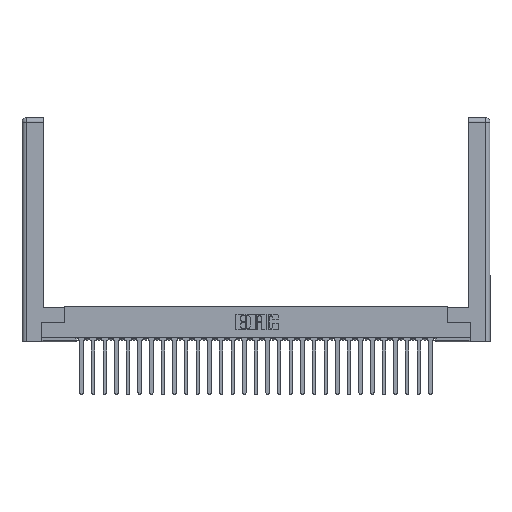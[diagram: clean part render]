
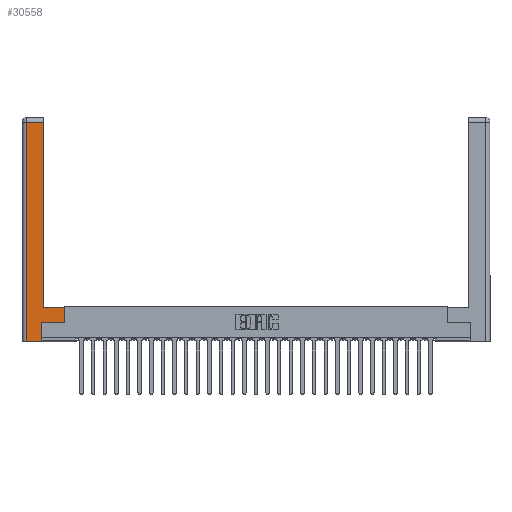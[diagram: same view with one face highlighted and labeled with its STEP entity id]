
A CAD part, top view. The second image highlights one B-rep face of the part: STEP entity #30558.
In plain terms, the highlighted planar face has unit normal (0, 0, 1).
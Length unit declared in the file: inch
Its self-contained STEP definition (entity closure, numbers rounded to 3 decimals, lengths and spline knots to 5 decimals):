
#816 = EDGE_CURVE ( 'NONE', #7851, #13557, #26790, .T. ) ;
#1370 = VECTOR ( 'NONE', #30396, 39.37008 ) ;
#1423 = LINE ( 'NONE', #20603, #13784 ) ;
#1588 = CARTESIAN_POINT ( 'NONE',  ( 0.565, 0.245, 0. ) ) ;
#1632 = EDGE_CURVE ( 'NONE', #27412, #3322, #6117, .T. ) ;
#2188 = CARTESIAN_POINT ( 'NONE',  ( 0.0615, 2.94, 0. ) ) ;
#3204 = VERTEX_POINT ( 'NONE', #18032 ) ;
#3322 = VERTEX_POINT ( 'NONE', #6363 ) ;
#3396 = EDGE_CURVE ( 'NONE', #24306, #16625, #15951, .T. ) ;
#3517 = VECTOR ( 'NONE', #18818, 39.37008 ) ;
#3655 = LINE ( 'NONE', #1588, #3517 ) ;
#4124 = CARTESIAN_POINT ( 'NONE',  ( 0.265, 0.245, 0. ) ) ;
#4247 = DIRECTION ( 'NONE',  ( -1., 0., 0. ) ) ;
#4993 = EDGE_CURVE ( 'NONE', #13557, #3204, #1423, .T. ) ;
#6117 = LINE ( 'NONE', #13631, #1370 ) ;
#6363 = CARTESIAN_POINT ( 'NONE',  ( 0.295, 0.45, 0. ) ) ;
#7851 = VERTEX_POINT ( 'NONE', #11325 ) ;
#9939 = CARTESIAN_POINT ( 'NONE',  ( 0.295, 3., 0. ) ) ;
#10257 = DIRECTION ( 'NONE',  ( 0., 1., 0. ) ) ;
#10413 = LINE ( 'NONE', #9939, #29787 ) ;
#11007 = EDGE_CURVE ( 'NONE', #3204, #24306, #26500, .T. ) ;
#11325 = CARTESIAN_POINT ( 'NONE',  ( 0.295, 2.94, 0. ) ) ;
#12130 = CARTESIAN_POINT ( 'NONE',  ( 0.265, 0., 0. ) ) ;
#12158 = VECTOR ( 'NONE', #16898, 39.37008 ) ;
#12792 = CARTESIAN_POINT ( 'NONE',  ( 0.565, 0.45, 0. ) ) ;
#13346 = ORIENTED_EDGE ( 'NONE', *, *, #23628, .T. ) ;
#13391 = EDGE_CURVE ( 'NONE', #21842, #27412, #25237, .T. ) ;
#13557 = VERTEX_POINT ( 'NONE', #30492 ) ;
#13631 = CARTESIAN_POINT ( 'NONE',  ( 0.295, 0.45, 0. ) ) ;
#13680 = CARTESIAN_POINT ( 'NONE',  ( 0., 0., 0. ) ) ;
#13784 = VECTOR ( 'NONE', #22851, 39.37008 ) ;
#13900 = ORIENTED_EDGE ( 'NONE', *, *, #816, .T. ) ;
#15951 = LINE ( 'NONE', #23307, #31507 ) ;
#16625 = VERTEX_POINT ( 'NONE', #4124 ) ;
#16898 = DIRECTION ( 'NONE',  ( 1., 0., 0. ) ) ;
#18032 = CARTESIAN_POINT ( 'NONE',  ( 0.0615, 0., 0. ) ) ;
#18551 = VECTOR ( 'NONE', #26313, 39.37008 ) ;
#18780 = DIRECTION ( 'NONE',  ( 0., 0., -1. ) ) ;
#18818 = DIRECTION ( 'NONE',  ( 1., 0., 0. ) ) ;
#18858 = ORIENTED_EDGE ( 'NONE', *, *, #11007, .T. ) ;
#19719 = EDGE_LOOP ( 'NONE', ( #13346, #13900, #30531, #18858, #31409, #21806, #28352, #22581 ) ) ;
#20603 = CARTESIAN_POINT ( 'NONE',  ( 0.0615, 0., 0. ) ) ;
#21181 = CARTESIAN_POINT ( 'NONE',  ( 0.265, 0., 0. ) ) ;
#21204 = FACE_OUTER_BOUND ( 'NONE', #19719, .T. ) ;
#21806 = ORIENTED_EDGE ( 'NONE', *, *, #30182, .T. ) ;
#21842 = VERTEX_POINT ( 'NONE', #22589 ) ;
#22581 = ORIENTED_EDGE ( 'NONE', *, *, #1632, .T. ) ;
#22589 = CARTESIAN_POINT ( 'NONE',  ( 0.565, 0.245, 0. ) ) ;
#22851 = DIRECTION ( 'NONE',  ( 0., -1., 0. ) ) ;
#23307 = CARTESIAN_POINT ( 'NONE',  ( 0.265, 0.245, 0. ) ) ;
#23628 = EDGE_CURVE ( 'NONE', #3322, #7851, #10413, .T. ) ;
#24306 = VERTEX_POINT ( 'NONE', #21181 ) ;
#25237 = LINE ( 'NONE', #12792, #26061 ) ;
#26061 = VECTOR ( 'NONE', #27321, 39.37008 ) ;
#26313 = DIRECTION ( 'NONE',  ( -1., 0., 0. ) ) ;
#26404 = AXIS2_PLACEMENT_3D ( 'NONE', #13680, #18780, #4247 ) ;
#26500 = LINE ( 'NONE', #12130, #12158 ) ;
#26790 = LINE ( 'NONE', #2188, #18551 ) ;
#27321 = DIRECTION ( 'NONE',  ( 0., 1., 0. ) ) ;
#27412 = VERTEX_POINT ( 'NONE', #30598 ) ;
#28352 = ORIENTED_EDGE ( 'NONE', *, *, #13391, .T. ) ;
#29787 = VECTOR ( 'NONE', #10257, 39.37008 ) ;
#30182 = EDGE_CURVE ( 'NONE', #16625, #21842, #3655, .T. ) ;
#30396 = DIRECTION ( 'NONE',  ( -1., 0., 0. ) ) ;
#30492 = CARTESIAN_POINT ( 'NONE',  ( 0.0615, 2.94, 0. ) ) ;
#30531 = ORIENTED_EDGE ( 'NONE', *, *, #4993, .T. ) ;
#30558 = ADVANCED_FACE ( 'NONE', ( #21204 ), #30922, .F. ) ;
#30598 = CARTESIAN_POINT ( 'NONE',  ( 0.565, 0.45, 0. ) ) ;
#30922 = PLANE ( 'NONE',  #26404 ) ;
#30955 = DIRECTION ( 'NONE',  ( 0., 1., 0. ) ) ;
#31409 = ORIENTED_EDGE ( 'NONE', *, *, #3396, .T. ) ;
#31507 = VECTOR ( 'NONE', #30955, 39.37008 ) ;
